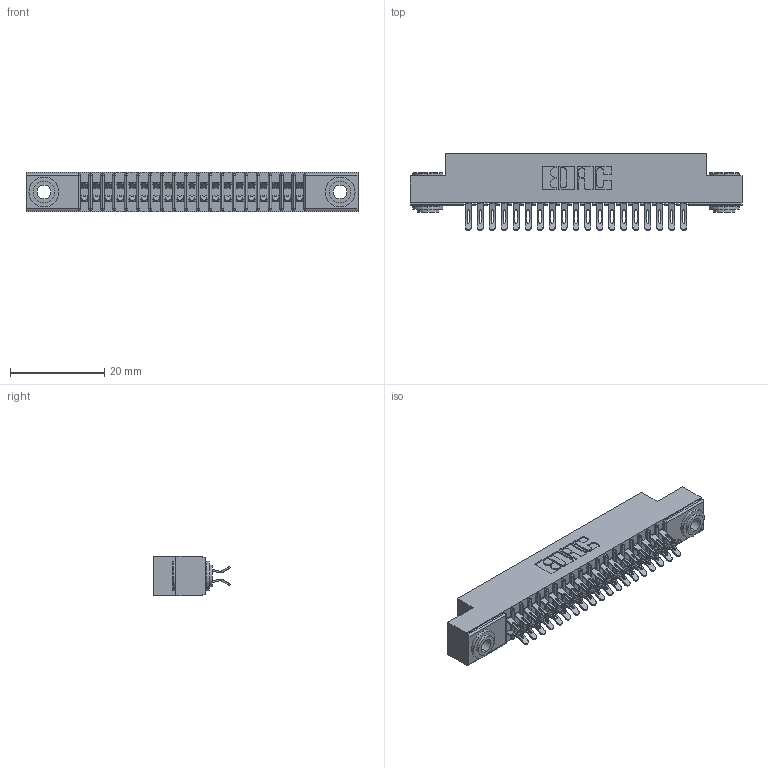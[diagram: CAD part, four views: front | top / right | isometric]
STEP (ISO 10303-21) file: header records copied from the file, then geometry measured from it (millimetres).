
FILE_DESCRIPTION (( 'STEP AP203' ), '1' );
FILE_NAME ('391-038-555-203.STEP', '2018-08-09T00:20:19', ( '' ), ( '' ), 'SwSTEP 2.0', 'SolidWorks 2016', '' );
FILE_SCHEMA (( 'CONFIG_CONTROL_DESIGN' ));
Length unit declared in the file: inch
Products named in the file (4): 391-038-555-203; 341 Part_.156 (3.96) Dia Mounting Holes; 341-292-001_341-292-155; 345-250-002_345-250-002-102
Assembly tree (41 placements, depth 2):
  391-038-555-203
    341 Part_.156 (3.96) Dia Mounting Holes
    341-292-001_341-292-155  x38
    345-250-002_345-250-002-102  x2
Bounding box: 70.48 x 16.31 x 8.38 mm (x, y, z)
Volume: 4070.6 mm3; surface area: 8832.5 mm2
Topology: 41 solids, 41 shells, 3132 faces, 9301 edges, 6054 vertices
Faces by surface type: plane 1688, cylinder 1360, sphere 40, torus 36, cone 8
Entity records: 27593 total; most frequent: CARTESIAN_POINT 4584, ORIENTED_EDGE 4534, DIRECTION 4471, EDGE_CURVE 2267, LINE 1781, VECTOR 1781, VERTEX_POINT 1442, AXIS2_PLACEMENT_3D 1345
